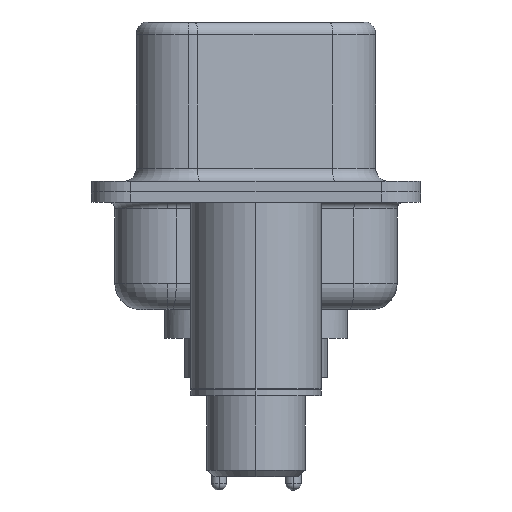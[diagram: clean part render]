
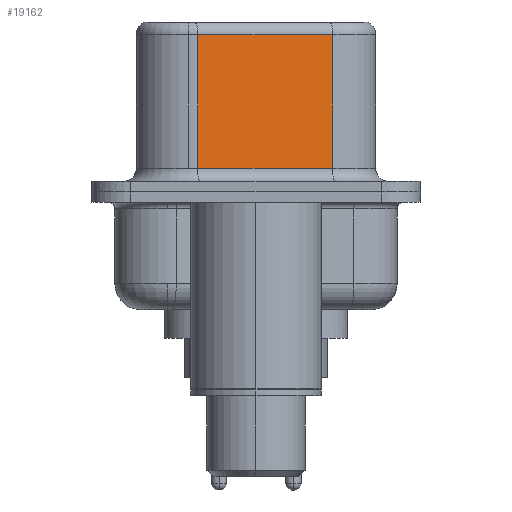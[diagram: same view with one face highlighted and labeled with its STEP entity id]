
A CAD part, left-side view. The second image highlights one B-rep face of the part: STEP entity #19162.
In plain terms, the highlighted planar face has unit normal (-0.985, -0.174, 0).
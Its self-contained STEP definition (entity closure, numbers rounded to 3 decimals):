
#677 = PLANE ( 'NONE',  #5162 ) ;
#802 = VERTEX_POINT ( 'NONE', #7402 ) ;
#2633 = DIRECTION ( 'NONE',  ( 0., 0., -1. ) ) ;
#3161 = ORIENTED_EDGE ( 'NONE', *, *, #5423, .T. ) ;
#3333 = CARTESIAN_POINT ( 'NONE',  ( 3.675, 2.233, 0.9 ) ) ;
#4265 = CARTESIAN_POINT ( 'NONE',  ( 4.585, -2.927, 6.02 ) ) ;
#4901 = VECTOR ( 'NONE', #15077, 1000. ) ;
#5102 = EDGE_CURVE ( 'NONE', #15000, #12488, #17249, .T. ) ;
#5162 = AXIS2_PLACEMENT_3D ( 'NONE', #16006, #14436, #8362 ) ;
#5169 = LINE ( 'NONE', #18042, #13143 ) ;
#5423 = EDGE_CURVE ( 'NONE', #12488, #17257, #8510, .T. ) ;
#7402 = CARTESIAN_POINT ( 'NONE',  ( 4.585, -2.927, 0.9 ) ) ;
#8362 = DIRECTION ( 'NONE',  ( -0.174, 0.985, 0. ) ) ;
#8510 = LINE ( 'NONE', #19613, #19175 ) ;
#9383 = DIRECTION ( 'NONE',  ( 0., 0., -1. ) ) ;
#9617 = ORIENTED_EDGE ( 'NONE', *, *, #5102, .T. ) ;
#11516 = CARTESIAN_POINT ( 'NONE',  ( 3.675, 2.233, 6.02 ) ) ;
#11891 = EDGE_CURVE ( 'NONE', #17257, #802, #5169, .T. ) ;
#12488 = VERTEX_POINT ( 'NONE', #11516 ) ;
#12622 = CARTESIAN_POINT ( 'NONE',  ( 4.585, -2.927, 6.52 ) ) ;
#13143 = VECTOR ( 'NONE', #14779, 1000. ) ;
#14436 = DIRECTION ( 'NONE',  ( 0.985, 0.174, 0. ) ) ;
#14779 = DIRECTION ( 'NONE',  ( 0.174, -0.985, 0. ) ) ;
#14896 = LINE ( 'NONE', #12622, #19726 ) ;
#15000 = VERTEX_POINT ( 'NONE', #19225 ) ;
#15077 = DIRECTION ( 'NONE',  ( -0.174, 0.985, 0. ) ) ;
#15955 = EDGE_LOOP ( 'NONE', ( #17444, #9617, #3161, #17649 ) ) ;
#16006 = CARTESIAN_POINT ( 'NONE',  ( 4.585, -2.927, 6.52 ) ) ;
#16227 = EDGE_CURVE ( 'NONE', #15000, #802, #14896, .T. ) ;
#17238 = FACE_OUTER_BOUND ( 'NONE', #15955, .T. ) ;
#17249 = LINE ( 'NONE', #4265, #4901 ) ;
#17257 = VERTEX_POINT ( 'NONE', #3333 ) ;
#17444 = ORIENTED_EDGE ( 'NONE', *, *, #16227, .F. ) ;
#17649 = ORIENTED_EDGE ( 'NONE', *, *, #11891, .T. ) ;
#18042 = CARTESIAN_POINT ( 'NONE',  ( 4.585, -2.927, 0.9 ) ) ;
#19162 = ADVANCED_FACE ( 'NONE', ( #17238 ), #677, .F. ) ;
#19175 = VECTOR ( 'NONE', #2633, 1000. ) ;
#19225 = CARTESIAN_POINT ( 'NONE',  ( 4.585, -2.927, 6.02 ) ) ;
#19613 = CARTESIAN_POINT ( 'NONE',  ( 3.675, 2.233, 6.52 ) ) ;
#19726 = VECTOR ( 'NONE', #9383, 1000. ) ;
